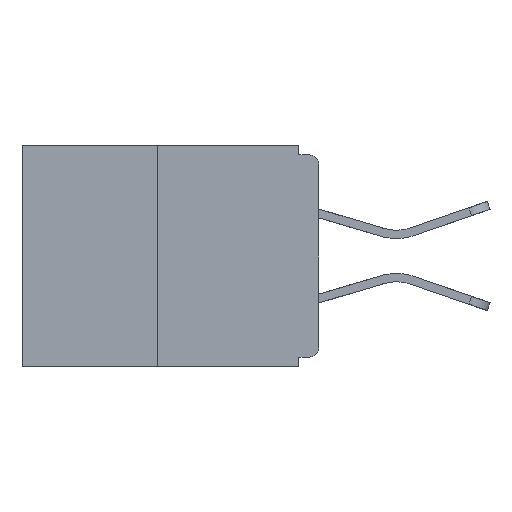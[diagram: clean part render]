
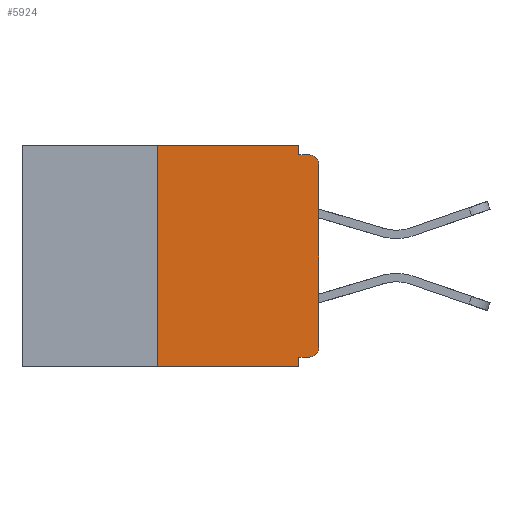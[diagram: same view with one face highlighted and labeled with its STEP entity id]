
A CAD part, left-side view. The second image highlights one B-rep face of the part: STEP entity #5924.
In plain terms, the highlighted planar face has unit normal (-1, 0, 0).
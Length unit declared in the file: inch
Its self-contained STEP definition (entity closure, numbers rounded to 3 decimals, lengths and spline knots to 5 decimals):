
#570 = VECTOR ( 'NONE', #15789, 39.37008 ) ;
#703 = DIRECTION ( 'NONE',  ( 0., 1., 0. ) ) ;
#812 = ORIENTED_EDGE ( 'NONE', *, *, #26716, .F. ) ;
#979 = CARTESIAN_POINT ( 'NONE',  ( 0., 0., 0. ) ) ;
#1202 = ORIENTED_EDGE ( 'NONE', *, *, #2922, .F. ) ;
#1256 = EDGE_CURVE ( 'NONE', #10443, #26148, #4722, .T. ) ;
#1743 = DIRECTION ( 'NONE',  ( 0., 0., -1. ) ) ;
#2680 = CARTESIAN_POINT ( 'NONE',  ( 0., 0.031, -0.343 ) ) ;
#2699 = CARTESIAN_POINT ( 'NONE',  ( 0., 0., -0.015 ) ) ;
#2772 = LINE ( 'NONE', #15515, #570 ) ;
#2831 = VERTEX_POINT ( 'NONE', #23893 ) ;
#2922 = EDGE_CURVE ( 'NONE', #14790, #2831, #13135, .T. ) ;
#3562 = VERTEX_POINT ( 'NONE', #18642 ) ;
#3683 = VECTOR ( 'NONE', #26591, 39.37008 ) ;
#3741 = EDGE_LOOP ( 'NONE', ( #1202, #6355, #11118, #11383, #12069, #4105, #23572, #4765, #14551, #812 ) ) ;
#4105 = ORIENTED_EDGE ( 'NONE', *, *, #4406, .T. ) ;
#4406 = EDGE_CURVE ( 'NONE', #13751, #10443, #15191, .T. ) ;
#4682 = VERTEX_POINT ( 'NONE', #12437 ) ;
#4722 = LINE ( 'NONE', #979, #12897 ) ;
#4765 = ORIENTED_EDGE ( 'NONE', *, *, #14252, .T. ) ;
#5151 = DIRECTION ( 'NONE',  ( 0., -1., 0. ) ) ;
#5504 = CARTESIAN_POINT ( 'NONE',  ( 0., 0.015, -0.328 ) ) ;
#5924 = ADVANCED_FACE ( 'NONE', ( #11465 ), #13609, .F. ) ;
#6355 = ORIENTED_EDGE ( 'NONE', *, *, #25978, .F. ) ;
#6583 = CARTESIAN_POINT ( 'NONE',  ( 0., 0.46, 0. ) ) ;
#6616 = CARTESIAN_POINT ( 'NONE',  ( 0., 0.015, -0.313 ) ) ;
#7494 = DIRECTION ( 'NONE',  ( 1., 0., 0. ) ) ;
#8111 = CIRCLE ( 'NONE', #13107, 0.015 ) ;
#8253 = DIRECTION ( 'NONE',  ( 0., 0., 1. ) ) ;
#8321 = LINE ( 'NONE', #19326, #25700 ) ;
#8369 = CARTESIAN_POINT ( 'NONE',  ( 0., 0., -0.313 ) ) ;
#8889 = DIRECTION ( 'NONE',  ( -1., 0., 0. ) ) ;
#9707 = LINE ( 'NONE', #2699, #22010 ) ;
#10313 = DIRECTION ( 'NONE',  ( 0., 0., -1. ) ) ;
#10443 = VERTEX_POINT ( 'NONE', #8369 ) ;
#11118 = ORIENTED_EDGE ( 'NONE', *, *, #12235, .T. ) ;
#11130 = EDGE_CURVE ( 'NONE', #13751, #20254, #26755, .T. ) ;
#11383 = ORIENTED_EDGE ( 'NONE', *, *, #21866, .F. ) ;
#11465 = FACE_OUTER_BOUND ( 'NONE', #3741, .T. ) ;
#11609 = CARTESIAN_POINT ( 'NONE',  ( 0., 0.46, 0. ) ) ;
#11798 = LINE ( 'NONE', #18407, #17969 ) ;
#12069 = ORIENTED_EDGE ( 'NONE', *, *, #11130, .F. ) ;
#12235 = EDGE_CURVE ( 'NONE', #4682, #22386, #2772, .T. ) ;
#12437 = CARTESIAN_POINT ( 'NONE',  ( 0., 0.25, -0.343 ) ) ;
#12897 = VECTOR ( 'NONE', #8253, 39.37008 ) ;
#13107 = AXIS2_PLACEMENT_3D ( 'NONE', #23189, #19183, #10313 ) ;
#13135 = LINE ( 'NONE', #6583, #3683 ) ;
#13354 = EDGE_CURVE ( 'NONE', #3562, #24655, #9707, .T. ) ;
#13609 = PLANE ( 'NONE',  #17729 ) ;
#13751 = VERTEX_POINT ( 'NONE', #5504 ) ;
#13761 = DIRECTION ( 'NONE',  ( 0., 0., -1. ) ) ;
#14252 = EDGE_CURVE ( 'NONE', #26148, #24655, #8111, .T. ) ;
#14551 = ORIENTED_EDGE ( 'NONE', *, *, #13354, .F. ) ;
#14790 = VERTEX_POINT ( 'NONE', #19151 ) ;
#15191 = CIRCLE ( 'NONE', #16546, 0.015 ) ;
#15336 = DIRECTION ( 'NONE',  ( 0., 0., -1. ) ) ;
#15449 = DIRECTION ( 'NONE',  ( 0., 0., 1. ) ) ;
#15515 = CARTESIAN_POINT ( 'NONE',  ( 0., 0.46, -0.343 ) ) ;
#15588 = VECTOR ( 'NONE', #703, 39.37008 ) ;
#15789 = DIRECTION ( 'NONE',  ( 0., -1., 0. ) ) ;
#16546 = AXIS2_PLACEMENT_3D ( 'NONE', #6616, #8889, #15336 ) ;
#16915 = CARTESIAN_POINT ( 'NONE',  ( 0., 0.031, -0.343 ) ) ;
#17729 = AXIS2_PLACEMENT_3D ( 'NONE', #11609, #7494, #13761 ) ;
#17781 = CARTESIAN_POINT ( 'NONE',  ( 0., 0.031, -0.328 ) ) ;
#17969 = VECTOR ( 'NONE', #24975, 39.37008 ) ;
#18407 = CARTESIAN_POINT ( 'NONE',  ( 0., 0.031, 0. ) ) ;
#18642 = CARTESIAN_POINT ( 'NONE',  ( 0., 0.031, -0.015 ) ) ;
#19151 = CARTESIAN_POINT ( 'NONE',  ( 0., 0.25, 0. ) ) ;
#19183 = DIRECTION ( 'NONE',  ( -1., 0., 0. ) ) ;
#19326 = CARTESIAN_POINT ( 'NONE',  ( 0., 0.25, 0. ) ) ;
#20254 = VERTEX_POINT ( 'NONE', #17781 ) ;
#21866 = EDGE_CURVE ( 'NONE', #20254, #22386, #23487, .T. ) ;
#22010 = VECTOR ( 'NONE', #5151, 39.37008 ) ;
#22155 = CARTESIAN_POINT ( 'NONE',  ( 0., 0., -0.03 ) ) ;
#22164 = CARTESIAN_POINT ( 'NONE',  ( 0., 0., -0.328 ) ) ;
#22386 = VERTEX_POINT ( 'NONE', #2680 ) ;
#23189 = CARTESIAN_POINT ( 'NONE',  ( 0., 0.015, -0.03 ) ) ;
#23487 = LINE ( 'NONE', #16915, #27475 ) ;
#23572 = ORIENTED_EDGE ( 'NONE', *, *, #1256, .T. ) ;
#23893 = CARTESIAN_POINT ( 'NONE',  ( 0., 0.031, 0. ) ) ;
#24655 = VERTEX_POINT ( 'NONE', #26188 ) ;
#24975 = DIRECTION ( 'NONE',  ( 0., 0., -1. ) ) ;
#25700 = VECTOR ( 'NONE', #15449, 39.37008 ) ;
#25978 = EDGE_CURVE ( 'NONE', #4682, #14790, #8321, .T. ) ;
#26148 = VERTEX_POINT ( 'NONE', #22155 ) ;
#26188 = CARTESIAN_POINT ( 'NONE',  ( 0., 0.015, -0.015 ) ) ;
#26591 = DIRECTION ( 'NONE',  ( 0., -1., 0. ) ) ;
#26716 = EDGE_CURVE ( 'NONE', #2831, #3562, #11798, .T. ) ;
#26755 = LINE ( 'NONE', #22164, #15588 ) ;
#27475 = VECTOR ( 'NONE', #1743, 39.37008 ) ;
